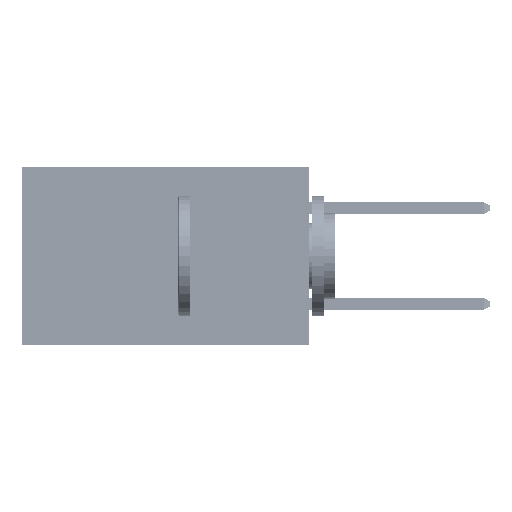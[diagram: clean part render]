
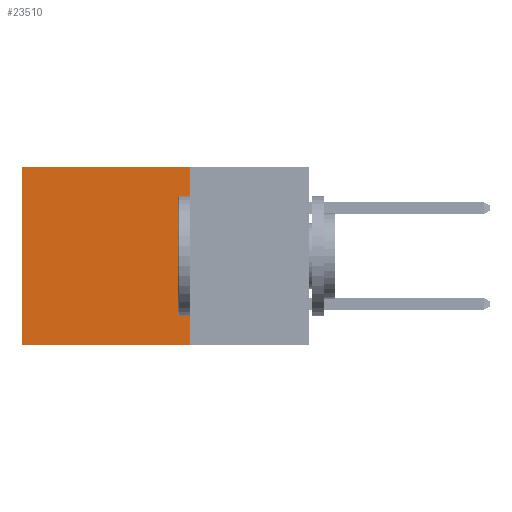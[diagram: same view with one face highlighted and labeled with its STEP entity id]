
A CAD part, left-side view. The second image highlights one B-rep face of the part: STEP entity #23510.
In plain terms, the highlighted planar face has unit normal (-1, 0, 0).
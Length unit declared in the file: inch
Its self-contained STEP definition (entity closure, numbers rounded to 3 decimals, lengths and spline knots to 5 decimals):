
#606 = VECTOR ( 'NONE', #8345, 39.37008 ) ;
#2282 = LINE ( 'NONE', #30782, #47505 ) ;
#5684 = VERTEX_POINT ( 'NONE', #33248 ) ;
#6385 = DIRECTION ( 'NONE',  ( 0., 0., -1. ) ) ;
#7451 = FACE_OUTER_BOUND ( 'NONE', #25870, .T. ) ;
#7804 = EDGE_CURVE ( 'NONE', #5684, #19897, #14317, .T. ) ;
#8004 = DIRECTION ( 'NONE',  ( 0., 1., 0. ) ) ;
#8345 = DIRECTION ( 'NONE',  ( 0., 0., -1. ) ) ;
#8398 = VERTEX_POINT ( 'NONE', #45804 ) ;
#9450 = VERTEX_POINT ( 'NONE', #39552 ) ;
#14317 = LINE ( 'NONE', #27262, #606 ) ;
#15966 = DIRECTION ( 'NONE',  ( 0., 0., -1. ) ) ;
#16726 = ORIENTED_EDGE ( 'NONE', *, *, #46080, .T. ) ;
#17679 = AXIS2_PLACEMENT_3D ( 'NONE', #42310, #47428, #6385 ) ;
#19612 = CARTESIAN_POINT ( 'NONE',  ( 0.2875, 0.25, -0.37 ) ) ;
#19729 = DIRECTION ( 'NONE',  ( 0., 1., 0. ) ) ;
#19897 = VERTEX_POINT ( 'NONE', #21117 ) ;
#21117 = CARTESIAN_POINT ( 'NONE',  ( 0.2875, 0.6, -0.37 ) ) ;
#23510 = ADVANCED_FACE ( 'NONE', ( #7451 ), #27047, .F. ) ;
#23610 = CARTESIAN_POINT ( 'NONE',  ( 0.2875, 0.25, 0. ) ) ;
#23854 = ORIENTED_EDGE ( 'NONE', *, *, #31409, .F. ) ;
#25371 = LINE ( 'NONE', #23610, #28928 ) ;
#25870 = EDGE_LOOP ( 'NONE', ( #31675, #44413, #23854, #16726 ) ) ;
#27047 = PLANE ( 'NONE',  #17679 ) ;
#27262 = CARTESIAN_POINT ( 'NONE',  ( 0.2875, 0.6, 0. ) ) ;
#28928 = VECTOR ( 'NONE', #15966, 39.37008 ) ;
#30559 = VECTOR ( 'NONE', #8004, 39.37008 ) ;
#30782 = CARTESIAN_POINT ( 'NONE',  ( 0.2875, 0.25, 0. ) ) ;
#31409 = EDGE_CURVE ( 'NONE', #8398, #9450, #25371, .T. ) ;
#31675 = ORIENTED_EDGE ( 'NONE', *, *, #7804, .T. ) ;
#33248 = CARTESIAN_POINT ( 'NONE',  ( 0.2875, 0.6, 0. ) ) ;
#35690 = EDGE_CURVE ( 'NONE', #9450, #19897, #44863, .T. ) ;
#39552 = CARTESIAN_POINT ( 'NONE',  ( 0.2875, 0.25, -0.37 ) ) ;
#42310 = CARTESIAN_POINT ( 'NONE',  ( 0.2875, 0.25, 0. ) ) ;
#44413 = ORIENTED_EDGE ( 'NONE', *, *, #35690, .F. ) ;
#44863 = LINE ( 'NONE', #19612, #30559 ) ;
#45804 = CARTESIAN_POINT ( 'NONE',  ( 0.2875, 0.25, 0. ) ) ;
#46080 = EDGE_CURVE ( 'NONE', #8398, #5684, #2282, .T. ) ;
#47428 = DIRECTION ( 'NONE',  ( 1., 0., 0. ) ) ;
#47505 = VECTOR ( 'NONE', #19729, 39.37008 ) ;
